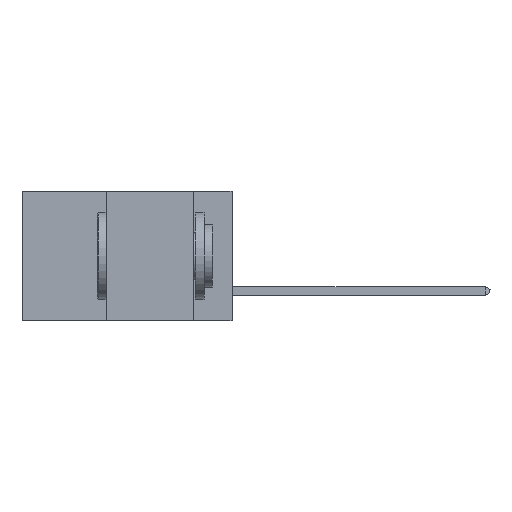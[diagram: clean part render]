
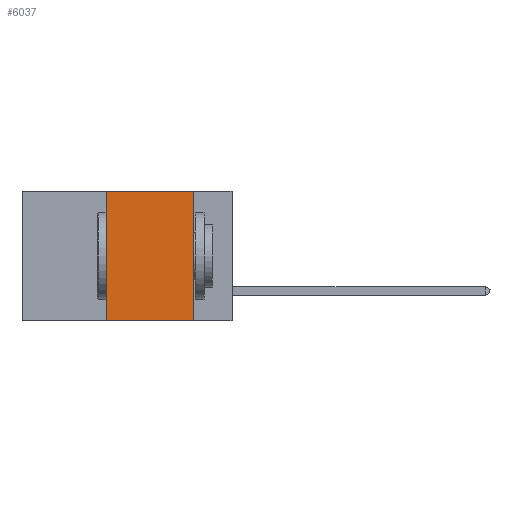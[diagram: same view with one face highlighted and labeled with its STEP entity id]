
A CAD part, left-side view. The second image highlights one B-rep face of the part: STEP entity #6037.
In plain terms, the highlighted planar face has unit normal (-1, 0, 0).
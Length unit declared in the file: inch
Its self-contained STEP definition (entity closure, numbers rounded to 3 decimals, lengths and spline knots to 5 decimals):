
#553 = VECTOR ( 'NONE', #15052, 39.37008 ) ;
#1859 = FACE_OUTER_BOUND ( 'NONE', #9036, .T. ) ;
#1908 = LINE ( 'NONE', #16395, #12914 ) ;
#1995 = DIRECTION ( 'NONE',  ( 0., 0., -1. ) ) ;
#3396 = CARTESIAN_POINT ( 'NONE',  ( 0., 0.6, 0. ) ) ;
#3473 = EDGE_CURVE ( 'NONE', #7910, #7961, #11412, .T. ) ;
#3833 = ORIENTED_EDGE ( 'NONE', *, *, #11145, .F. ) ;
#4343 = VERTEX_POINT ( 'NONE', #16931 ) ;
#4418 = LINE ( 'NONE', #12130, #11598 ) ;
#5013 = CARTESIAN_POINT ( 'NONE',  ( 0., 0.6, -0.37 ) ) ;
#5029 = DIRECTION ( 'NONE',  ( 0., -1., 0. ) ) ;
#5240 = VERTEX_POINT ( 'NONE', #17753 ) ;
#6037 = ADVANCED_FACE ( 'NONE', ( #1859 ), #18514, .F. ) ;
#6995 = DIRECTION ( 'NONE',  ( 0., 0., -1. ) ) ;
#7071 = ORIENTED_EDGE ( 'NONE', *, *, #3473, .T. ) ;
#7182 = DIRECTION ( 'NONE',  ( 1., 0., 0. ) ) ;
#7805 = DIRECTION ( 'NONE',  ( 0., 0., 1. ) ) ;
#7910 = VERTEX_POINT ( 'NONE', #14710 ) ;
#7961 = VERTEX_POINT ( 'NONE', #17628 ) ;
#7976 = AXIS2_PLACEMENT_3D ( 'NONE', #14138, #7182, #6995 ) ;
#8423 = ORIENTED_EDGE ( 'NONE', *, *, #17533, .F. ) ;
#9036 = EDGE_LOOP ( 'NONE', ( #16116, #8423, #3833, #7071 ) ) ;
#11145 = EDGE_CURVE ( 'NONE', #7910, #4343, #1908, .T. ) ;
#11195 = EDGE_CURVE ( 'NONE', #5240, #7961, #4418, .T. ) ;
#11384 = VECTOR ( 'NONE', #5029, 39.37008 ) ;
#11412 = LINE ( 'NONE', #5013, #553 ) ;
#11598 = VECTOR ( 'NONE', #1995, 39.37008 ) ;
#12130 = CARTESIAN_POINT ( 'NONE',  ( 0., 0.11, 0. ) ) ;
#12914 = VECTOR ( 'NONE', #7805, 39.37008 ) ;
#14138 = CARTESIAN_POINT ( 'NONE',  ( 0., 0.6, 0. ) ) ;
#14291 = LINE ( 'NONE', #3396, #11384 ) ;
#14710 = CARTESIAN_POINT ( 'NONE',  ( 0., 0.36, -0.37 ) ) ;
#15052 = DIRECTION ( 'NONE',  ( 0., -1., 0. ) ) ;
#16116 = ORIENTED_EDGE ( 'NONE', *, *, #11195, .F. ) ;
#16395 = CARTESIAN_POINT ( 'NONE',  ( 0., 0.36, 0. ) ) ;
#16931 = CARTESIAN_POINT ( 'NONE',  ( 0., 0.36, 0. ) ) ;
#17533 = EDGE_CURVE ( 'NONE', #4343, #5240, #14291, .T. ) ;
#17628 = CARTESIAN_POINT ( 'NONE',  ( 0., 0.11, -0.37 ) ) ;
#17753 = CARTESIAN_POINT ( 'NONE',  ( 0., 0.11, 0. ) ) ;
#18514 = PLANE ( 'NONE',  #7976 ) ;
